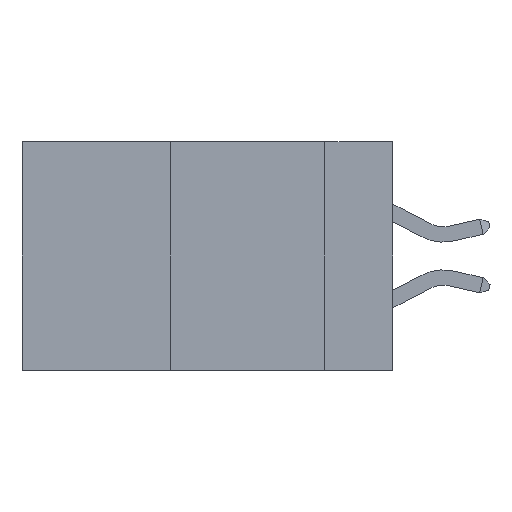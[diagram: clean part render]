
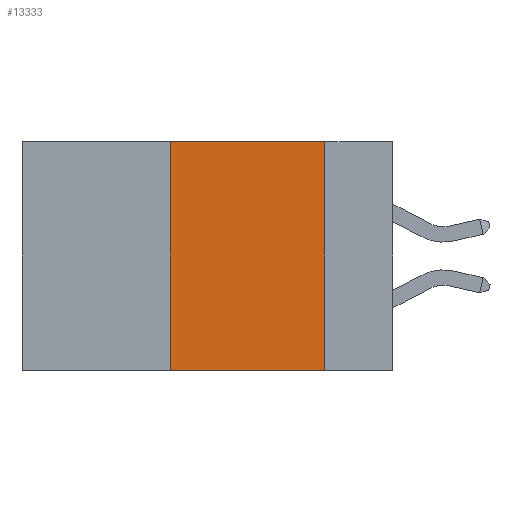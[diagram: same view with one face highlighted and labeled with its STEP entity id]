
A CAD part, left-side view. The second image highlights one B-rep face of the part: STEP entity #13333.
In plain terms, the highlighted planar face has unit normal (-1, 0, 0).
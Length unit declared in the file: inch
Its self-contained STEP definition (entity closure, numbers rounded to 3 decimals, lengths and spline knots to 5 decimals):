
#455 = PLANE ( 'NONE',  #10590 ) ;
#709 = LINE ( 'NONE', #3331, #4211 ) ;
#1108 = EDGE_CURVE ( 'NONE', #9645, #4842, #6090, .T. ) ;
#1151 = VECTOR ( 'NONE', #6613, 39.37008 ) ;
#2209 = EDGE_LOOP ( 'NONE', ( #11060, #9033, #8236, #4805 ) ) ;
#2312 = LINE ( 'NONE', #11941, #1151 ) ;
#2840 = VERTEX_POINT ( 'NONE', #13067 ) ;
#3125 = VECTOR ( 'NONE', #11363, 39.37008 ) ;
#3201 = CARTESIAN_POINT ( 'NONE',  ( 0., 0.6, -0.37 ) ) ;
#3331 = CARTESIAN_POINT ( 'NONE',  ( 0., 0.6, 0. ) ) ;
#3665 = CARTESIAN_POINT ( 'NONE',  ( 0., 0.6, 0. ) ) ;
#3803 = DIRECTION ( 'NONE',  ( 0., 0., -1. ) ) ;
#4211 = VECTOR ( 'NONE', #4532, 39.37008 ) ;
#4386 = FACE_OUTER_BOUND ( 'NONE', #2209, .T. ) ;
#4532 = DIRECTION ( 'NONE',  ( 0., -1., 0. ) ) ;
#4805 = ORIENTED_EDGE ( 'NONE', *, *, #1108, .T. ) ;
#4811 = CARTESIAN_POINT ( 'NONE',  ( 0., 0.11, -0.37 ) ) ;
#4842 = VERTEX_POINT ( 'NONE', #4811 ) ;
#5745 = EDGE_CURVE ( 'NONE', #2840, #4842, #7091, .T. ) ;
#6090 = LINE ( 'NONE', #3201, #11376 ) ;
#6613 = DIRECTION ( 'NONE',  ( 0., 0., 1. ) ) ;
#7091 = LINE ( 'NONE', #11310, #3125 ) ;
#8236 = ORIENTED_EDGE ( 'NONE', *, *, #11196, .F. ) ;
#8932 = EDGE_CURVE ( 'NONE', #12013, #2840, #709, .T. ) ;
#9033 = ORIENTED_EDGE ( 'NONE', *, *, #8932, .F. ) ;
#9597 = CARTESIAN_POINT ( 'NONE',  ( 0., 0.36, 0. ) ) ;
#9645 = VERTEX_POINT ( 'NONE', #11404 ) ;
#10590 = AXIS2_PLACEMENT_3D ( 'NONE', #3665, #12362, #3803 ) ;
#10897 = DIRECTION ( 'NONE',  ( 0., -1., 0. ) ) ;
#11060 = ORIENTED_EDGE ( 'NONE', *, *, #5745, .F. ) ;
#11196 = EDGE_CURVE ( 'NONE', #9645, #12013, #2312, .T. ) ;
#11310 = CARTESIAN_POINT ( 'NONE',  ( 0., 0.11, 0. ) ) ;
#11363 = DIRECTION ( 'NONE',  ( 0., 0., -1. ) ) ;
#11376 = VECTOR ( 'NONE', #10897, 39.37008 ) ;
#11404 = CARTESIAN_POINT ( 'NONE',  ( 0., 0.36, -0.37 ) ) ;
#11941 = CARTESIAN_POINT ( 'NONE',  ( 0., 0.36, 0. ) ) ;
#12013 = VERTEX_POINT ( 'NONE', #9597 ) ;
#12362 = DIRECTION ( 'NONE',  ( 1., 0., 0. ) ) ;
#13067 = CARTESIAN_POINT ( 'NONE',  ( 0., 0.11, 0. ) ) ;
#13333 = ADVANCED_FACE ( 'NONE', ( #4386 ), #455, .F. ) ;
